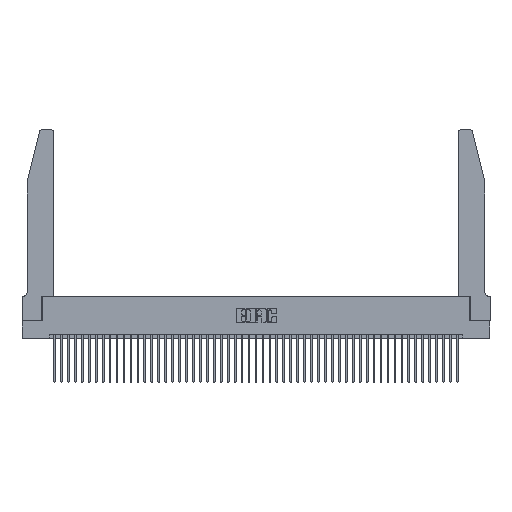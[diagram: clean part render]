
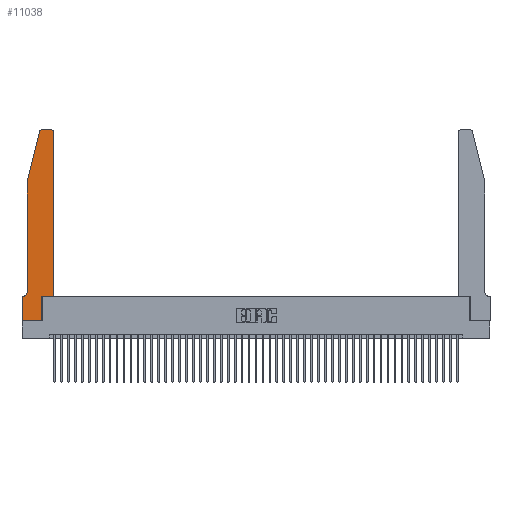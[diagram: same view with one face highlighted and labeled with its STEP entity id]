
A CAD part, top view. The second image highlights one B-rep face of the part: STEP entity #11038.
In plain terms, the highlighted planar face has unit normal (0, 0, 1).
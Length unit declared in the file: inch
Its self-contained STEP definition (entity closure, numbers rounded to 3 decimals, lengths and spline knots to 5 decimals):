
#313 = LINE ( 'NONE', #28895, #39339 ) ;
#650 = VERTEX_POINT ( 'NONE', #11244 ) ;
#807 = CIRCLE ( 'NONE', #12107, 0.03 ) ;
#1155 = EDGE_CURVE ( 'NONE', #27493, #48383, #4347, .T. ) ;
#2197 = DIRECTION ( 'NONE',  ( 0., -1., 0. ) ) ;
#2238 = DIRECTION ( 'NONE',  ( 1., 0., 0. ) ) ;
#2349 = CARTESIAN_POINT ( 'NONE',  ( 0.2865, 0., 0.37 ) ) ;
#2399 = ORIENTED_EDGE ( 'NONE', *, *, #24597, .T. ) ;
#2413 = DIRECTION ( 'NONE',  ( 0., -1., 0. ) ) ;
#2776 = VECTOR ( 'NONE', #2197, 39.37008 ) ;
#3134 = AXIS2_PLACEMENT_3D ( 'NONE', #5452, #31899, #9253 ) ;
#3639 = DIRECTION ( 'NONE',  ( -1., 0., 0. ) ) ;
#4335 = CIRCLE ( 'NONE', #7724, 0.07 ) ;
#4347 = LINE ( 'NONE', #40153, #23302 ) ;
#4445 = CARTESIAN_POINT ( 'NONE',  ( 0.0055, 0.35, 0.37 ) ) ;
#5452 = CARTESIAN_POINT ( 'NONE',  ( 0.284, 2.72, 0.37 ) ) ;
#5702 = AXIS2_PLACEMENT_3D ( 'NONE', #12876, #39210, #16688 ) ;
#6238 = VERTEX_POINT ( 'NONE', #38187 ) ;
#7055 = CARTESIAN_POINT ( 'NONE',  ( 0.4505, 0.35, 0.37 ) ) ;
#7724 = AXIS2_PLACEMENT_3D ( 'NONE', #48647, #26315, #3639 ) ;
#8551 = CARTESIAN_POINT ( 'NONE',  ( 0.284, 2.75, 0.37 ) ) ;
#9253 = DIRECTION ( 'NONE',  ( 1., 0., 0. ) ) ;
#9431 = DIRECTION ( 'NONE',  ( -0.239, -0.971, 0. ) ) ;
#9527 = ORIENTED_EDGE ( 'NONE', *, *, #15841, .T. ) ;
#9601 = DIRECTION ( 'NONE',  ( -1., 0., 0. ) ) ;
#9881 = CARTESIAN_POINT ( 'NONE',  ( 0., 0., 0.37 ) ) ;
#9937 = EDGE_LOOP ( 'NONE', ( #2399, #24934, #26134, #47121, #28481, #9527, #21995, #41924, #24353, #25548, #16000, #38361 ) ) ;
#10827 = LINE ( 'NONE', #15157, #22087 ) ;
#11038 = ADVANCED_FACE ( 'NONE', ( #40249 ), #35440, .T. ) ;
#11045 = EDGE_CURVE ( 'NONE', #13468, #41958, #30362, .T. ) ;
#11244 = CARTESIAN_POINT ( 'NONE',  ( 0., 0.35, 0.37 ) ) ;
#11257 = VECTOR ( 'NONE', #9431, 39.37008 ) ;
#12107 = AXIS2_PLACEMENT_3D ( 'NONE', #41534, #19047, #45276 ) ;
#12876 = CARTESIAN_POINT ( 'NONE',  ( 0., 0.35, 0.37 ) ) ;
#13468 = VERTEX_POINT ( 'NONE', #8551 ) ;
#13470 = CARTESIAN_POINT ( 'NONE',  ( 0.0755, 2., 0.37 ) ) ;
#13770 = LINE ( 'NONE', #36591, #32690 ) ;
#15157 = CARTESIAN_POINT ( 'NONE',  ( 0.4505, 0.35, 0.37 ) ) ;
#15841 = EDGE_CURVE ( 'NONE', #40838, #650, #29833, .T. ) ;
#16000 = ORIENTED_EDGE ( 'NONE', *, *, #48482, .T. ) ;
#16113 = EDGE_CURVE ( 'NONE', #18410, #40838, #4335, .T. ) ;
#16465 = LINE ( 'NONE', #9881, #34170 ) ;
#16688 = DIRECTION ( 'NONE',  ( 1., 0., 0. ) ) ;
#17394 = VECTOR ( 'NONE', #9601, 39.37008 ) ;
#17713 = EDGE_CURVE ( 'NONE', #44624, #27493, #24905, .T. ) ;
#18410 = VERTEX_POINT ( 'NONE', #38391 ) ;
#19047 = DIRECTION ( 'NONE',  ( 0., 0., 1. ) ) ;
#20031 = VERTEX_POINT ( 'NONE', #38764 ) ;
#20161 = EDGE_CURVE ( 'NONE', #41958, #6238, #21321, .T. ) ;
#21321 = LINE ( 'NONE', #43114, #11257 ) ;
#21924 = CARTESIAN_POINT ( 'NONE',  ( 0.25487, 2.72718, 0.37 ) ) ;
#21995 = ORIENTED_EDGE ( 'NONE', *, *, #43984, .T. ) ;
#22087 = VECTOR ( 'NONE', #26398, 39.37008 ) ;
#23207 = CARTESIAN_POINT ( 'NONE',  ( 0.2865, 0.35, 0.37 ) ) ;
#23302 = VECTOR ( 'NONE', #32684, 39.37008 ) ;
#24353 = ORIENTED_EDGE ( 'NONE', *, *, #17713, .T. ) ;
#24597 = EDGE_CURVE ( 'NONE', #20031, #13468, #13770, .T. ) ;
#24905 = LINE ( 'NONE', #23207, #43591 ) ;
#24934 = ORIENTED_EDGE ( 'NONE', *, *, #11045, .T. ) ;
#25140 = CARTESIAN_POINT ( 'NONE',  ( 0., 0., 0.37 ) ) ;
#25392 = VERTEX_POINT ( 'NONE', #44674 ) ;
#25548 = ORIENTED_EDGE ( 'NONE', *, *, #1155, .T. ) ;
#26134 = ORIENTED_EDGE ( 'NONE', *, *, #20161, .T. ) ;
#26315 = DIRECTION ( 'NONE',  ( 0., 0., -1. ) ) ;
#26398 = DIRECTION ( 'NONE',  ( 0., 1., 0. ) ) ;
#27493 = VERTEX_POINT ( 'NONE', #32081 ) ;
#28465 = CARTESIAN_POINT ( 'NONE',  ( 0.0755, 0.35, 0.37 ) ) ;
#28481 = ORIENTED_EDGE ( 'NONE', *, *, #16113, .T. ) ;
#28895 = CARTESIAN_POINT ( 'NONE',  ( 0., 0., 0.37 ) ) ;
#29418 = LINE ( 'NONE', #13470, #2776 ) ;
#29833 = LINE ( 'NONE', #28465, #17394 ) ;
#30362 = CIRCLE ( 'NONE', #3134, 0.03 ) ;
#31899 = DIRECTION ( 'NONE',  ( 0., 0., 1. ) ) ;
#32081 = CARTESIAN_POINT ( 'NONE',  ( 0.2865, 0.35, 0.37 ) ) ;
#32684 = DIRECTION ( 'NONE',  ( 1., 0., 0. ) ) ;
#32690 = VECTOR ( 'NONE', #32870, 39.37008 ) ;
#32870 = DIRECTION ( 'NONE',  ( -1., 0., 0. ) ) ;
#34170 = VECTOR ( 'NONE', #2238, 39.37008 ) ;
#35440 = PLANE ( 'NONE',  #5702 ) ;
#36591 = CARTESIAN_POINT ( 'NONE',  ( 0.2605, 2.75, 0.37 ) ) ;
#38187 = CARTESIAN_POINT ( 'NONE',  ( 0.0755, 2., 0.37 ) ) ;
#38361 = ORIENTED_EDGE ( 'NONE', *, *, #47176, .T. ) ;
#38391 = CARTESIAN_POINT ( 'NONE',  ( 0.0755, 0.42, 0.37 ) ) ;
#38764 = CARTESIAN_POINT ( 'NONE',  ( 0.4205, 2.75, 0.37 ) ) ;
#39210 = DIRECTION ( 'NONE',  ( 0., 0., 1. ) ) ;
#39339 = VECTOR ( 'NONE', #2413, 39.37008 ) ;
#40153 = CARTESIAN_POINT ( 'NONE',  ( 0.4505, 0.35, 0.37 ) ) ;
#40249 = FACE_OUTER_BOUND ( 'NONE', #9937, .T. ) ;
#40838 = VERTEX_POINT ( 'NONE', #4445 ) ;
#41534 = CARTESIAN_POINT ( 'NONE',  ( 0.4205, 2.72, 0.37 ) ) ;
#41924 = ORIENTED_EDGE ( 'NONE', *, *, #45844, .T. ) ;
#41958 = VERTEX_POINT ( 'NONE', #21924 ) ;
#43114 = CARTESIAN_POINT ( 'NONE',  ( 0.0755, 2., 0.37 ) ) ;
#43591 = VECTOR ( 'NONE', #45598, 39.37008 ) ;
#43984 = EDGE_CURVE ( 'NONE', #650, #47606, #313, .T. ) ;
#44624 = VERTEX_POINT ( 'NONE', #2349 ) ;
#44674 = CARTESIAN_POINT ( 'NONE',  ( 0.4505, 2.72, 0.37 ) ) ;
#45276 = DIRECTION ( 'NONE',  ( 1., 0., 0. ) ) ;
#45598 = DIRECTION ( 'NONE',  ( 0., 1., 0. ) ) ;
#45844 = EDGE_CURVE ( 'NONE', #47606, #44624, #16465, .T. ) ;
#46450 = EDGE_CURVE ( 'NONE', #6238, #18410, #29418, .T. ) ;
#47121 = ORIENTED_EDGE ( 'NONE', *, *, #46450, .T. ) ;
#47176 = EDGE_CURVE ( 'NONE', #25392, #20031, #807, .T. ) ;
#47606 = VERTEX_POINT ( 'NONE', #25140 ) ;
#48383 = VERTEX_POINT ( 'NONE', #7055 ) ;
#48482 = EDGE_CURVE ( 'NONE', #48383, #25392, #10827, .T. ) ;
#48647 = CARTESIAN_POINT ( 'NONE',  ( 0.0055, 0.42, 0.37 ) ) ;
